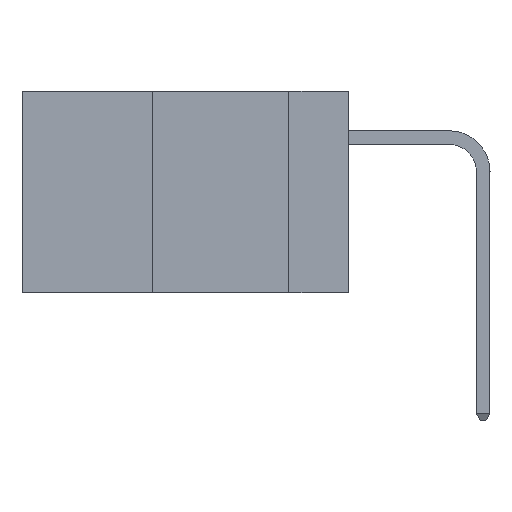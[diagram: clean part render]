
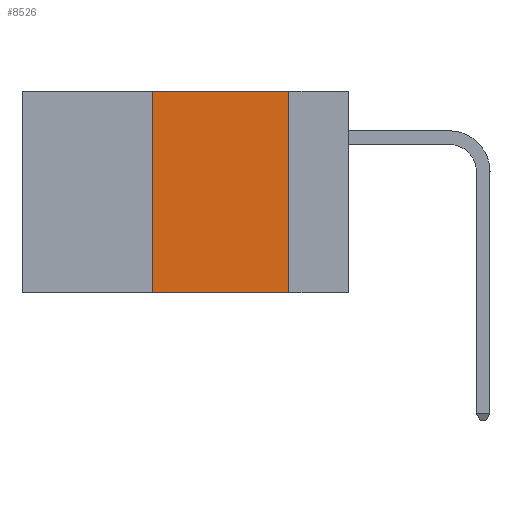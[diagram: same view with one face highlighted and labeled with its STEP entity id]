
A CAD part, left-side view. The second image highlights one B-rep face of the part: STEP entity #8526.
In plain terms, the highlighted planar face has unit normal (-1, 0, 0).
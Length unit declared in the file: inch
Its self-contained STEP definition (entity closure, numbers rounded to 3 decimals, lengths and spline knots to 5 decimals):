
#382 = EDGE_CURVE ( 'NONE', #6969, #2197, #6660, .T. ) ;
#399 = CARTESIAN_POINT ( 'NONE',  ( 0., 0.36, 0. ) ) ;
#400 = EDGE_CURVE ( 'NONE', #15719, #11020, #16979, .T. ) ;
#785 = PLANE ( 'NONE',  #7523 ) ;
#1005 = LINE ( 'NONE', #5434, #11547 ) ;
#1357 = DIRECTION ( 'NONE',  ( 0., 0., 1. ) ) ;
#1545 = CARTESIAN_POINT ( 'NONE',  ( 0., 0.6, 0. ) ) ;
#1861 = CARTESIAN_POINT ( 'NONE',  ( 0., 0.11, 0. ) ) ;
#2173 = DIRECTION ( 'NONE',  ( 1., 0., 0. ) ) ;
#2197 = VERTEX_POINT ( 'NONE', #1861 ) ;
#2468 = FACE_OUTER_BOUND ( 'NONE', #7361, .T. ) ;
#3171 = VECTOR ( 'NONE', #4086, 39.37008 ) ;
#3877 = DIRECTION ( 'NONE',  ( 0., -1., 0. ) ) ;
#4013 = CARTESIAN_POINT ( 'NONE',  ( 0., 0.11, 0. ) ) ;
#4086 = DIRECTION ( 'NONE',  ( 0., -1., 0. ) ) ;
#4572 = ORIENTED_EDGE ( 'NONE', *, *, #7552, .F. ) ;
#5434 = CARTESIAN_POINT ( 'NONE',  ( 0., 0.36, 0. ) ) ;
#5841 = CARTESIAN_POINT ( 'NONE',  ( 0., 0.36, -0.37 ) ) ;
#6660 = LINE ( 'NONE', #1545, #3171 ) ;
#6704 = ORIENTED_EDGE ( 'NONE', *, *, #400, .T. ) ;
#6969 = VERTEX_POINT ( 'NONE', #399 ) ;
#7361 = EDGE_LOOP ( 'NONE', ( #13745, #16551, #4572, #6704 ) ) ;
#7523 = AXIS2_PLACEMENT_3D ( 'NONE', #11319, #2173, #11374 ) ;
#7552 = EDGE_CURVE ( 'NONE', #15719, #6969, #1005, .T. ) ;
#8526 = ADVANCED_FACE ( 'NONE', ( #2468 ), #785, .F. ) ;
#8636 = VECTOR ( 'NONE', #13139, 39.37008 ) ;
#9157 = CARTESIAN_POINT ( 'NONE',  ( 0., 0.11, -0.37 ) ) ;
#9769 = VECTOR ( 'NONE', #3877, 39.37008 ) ;
#11020 = VERTEX_POINT ( 'NONE', #9157 ) ;
#11319 = CARTESIAN_POINT ( 'NONE',  ( 0., 0.6, 0. ) ) ;
#11374 = DIRECTION ( 'NONE',  ( 0., 0., -1. ) ) ;
#11547 = VECTOR ( 'NONE', #1357, 39.37008 ) ;
#11689 = LINE ( 'NONE', #4013, #8636 ) ;
#13139 = DIRECTION ( 'NONE',  ( 0., 0., -1. ) ) ;
#13745 = ORIENTED_EDGE ( 'NONE', *, *, #14785, .F. ) ;
#14785 = EDGE_CURVE ( 'NONE', #2197, #11020, #11689, .T. ) ;
#15670 = CARTESIAN_POINT ( 'NONE',  ( 0., 0.6, -0.37 ) ) ;
#15719 = VERTEX_POINT ( 'NONE', #5841 ) ;
#16551 = ORIENTED_EDGE ( 'NONE', *, *, #382, .F. ) ;
#16979 = LINE ( 'NONE', #15670, #9769 ) ;
